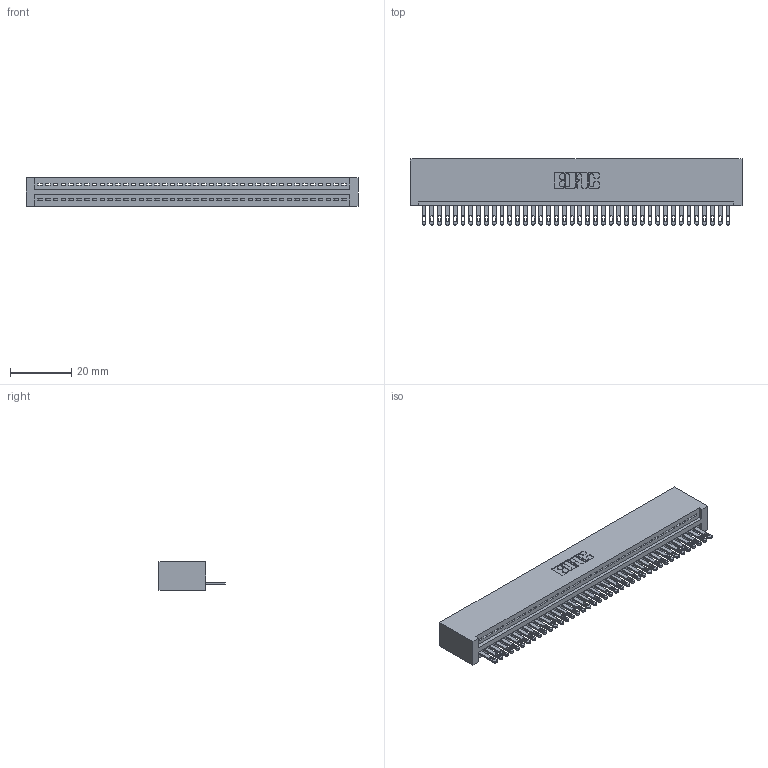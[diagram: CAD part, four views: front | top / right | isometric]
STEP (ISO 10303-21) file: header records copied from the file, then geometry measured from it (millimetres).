
FILE_DESCRIPTION (( 'STEP AP203' ), '1' );
FILE_NAME ('345-040-500-101.STEP', '2019-10-08T07:52:35', ( '' ), ( '' ), 'SwSTEP 2.0', 'SolidWorks 2016', '' );
FILE_SCHEMA (( 'CONFIG_CONTROL_DESIGN' ));
Length unit declared in the file: inch
Products named in the file (3): 345-040-500-101; 345-292-001_345-293-100; 345 Part_No Mounting Lugs
Assembly tree (41 placements, depth 2):
  345-040-500-101
    345 Part_No Mounting Lugs
    345-292-001_345-293-100  x40
Bounding box: 108.2 x 21.51 x 9.4 mm (x, y, z)
Volume: 10870.1 mm3; surface area: 14698.1 mm2
Topology: 41 solids, 41 shells, 2278 faces, 7037 edges, 4690 vertices
Faces by surface type: plane 1436, cylinder 842
Entity records: 30027 total; most frequent: CARTESIAN_POINT 5208, ORIENTED_EDGE 5182, DIRECTION 4547, EDGE_CURVE 2591, VECTOR 2303, LINE 2303, VERTEX_POINT 1726, AXIS2_PLACEMENT_3D 1122
